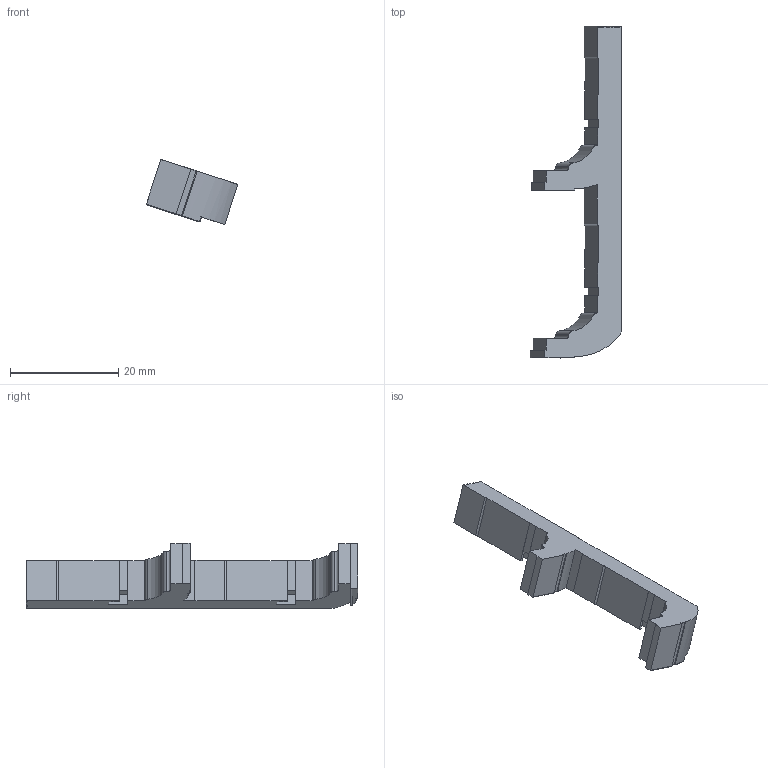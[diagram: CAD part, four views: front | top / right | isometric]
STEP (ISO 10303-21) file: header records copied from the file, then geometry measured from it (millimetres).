
FILE_DESCRIPTION(/* description */ (''),/* implementation_level */ '2;1');
FILE_NAME(/* name */ 'Glocknofsky Mag Release final.step',/* time_stamp */ '2022-04-02T15:38:10-04:00',/* author */ (''),/* organization */ (''),/* preprocessor_version */ 'ST-DEVELOPER v18.1',/* originating_system */ 'Autodesk Translation Framework v10.14.0.1471',/* authorisation */ '');
FILE_SCHEMA (('AUTOMOTIVE_DESIGN { 1 0 10303 214 3 1 1 }'));
Length unit declared in the file: millimetre
Products named in the file (1): modded mag release
Bounding box: 16.92 x 61.3 x 12.03 mm (x, y, z)
Volume: 2872.2 mm3; surface area: 2100.5 mm2
Topology: 1 solids, 1 shells, 86 faces, 246 edges, 162 vertices
Faces by surface type: plane 58, cylinder 23, torus 4, bspline 1
Entity records: 2965 total; most frequent: CARTESIAN_POINT 655, ORIENTED_EDGE 492, DIRECTION 466, EDGE_CURVE 246, LINE 190, VECTOR 190, VERTEX_POINT 162, AXIS2_PLACEMENT_3D 138
